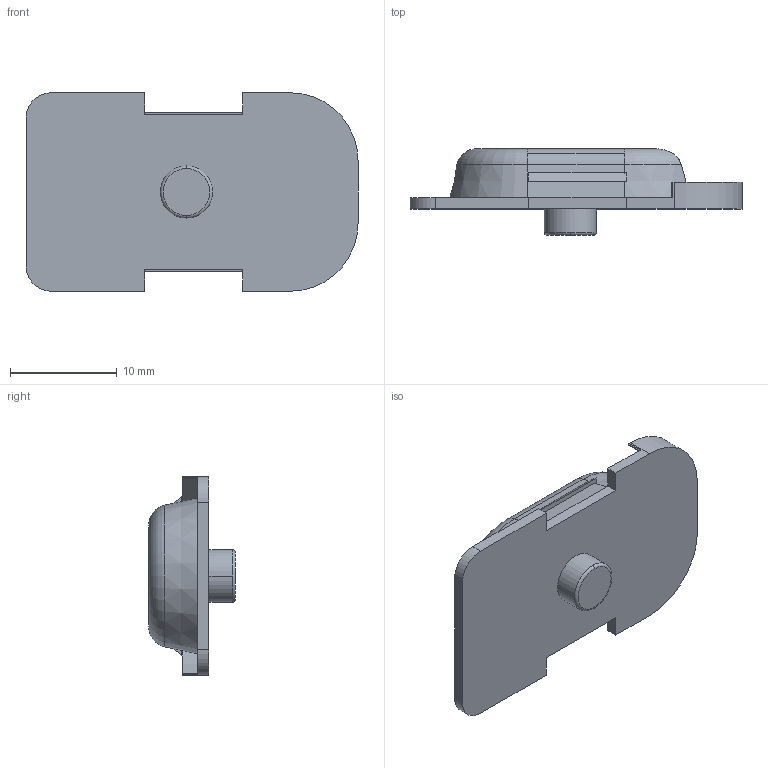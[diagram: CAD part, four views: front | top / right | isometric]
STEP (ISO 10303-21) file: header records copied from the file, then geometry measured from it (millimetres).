
FILE_DESCRIPTION (( 'STEP AP214' ), '1' );
FILE_NAME ('Magazine Insert.step', '2014-07-30T19:46:14', ( 'WarFairy' ), ( '' ), 'SwSTEP 2.0', 'SolidWorks 2013', '' );
FILE_SCHEMA (( 'AUTOMOTIVE_DESIGN' ));
Length unit declared in the file: millimetre
Products named in the file (1): Magazine Insert
Bounding box: 31.1 x 8.1 x 18.59 mm (x, y, z)
Volume: 1309.1 mm3; surface area: 1661.6 mm2
Topology: 1 solids, 1 shells, 70 faces, 189 edges, 122 vertices
Faces by surface type: plane 45, cylinder 18, torus 5, cone 2
Entity records: 2244 total; most frequent: CARTESIAN_POINT 412, DIRECTION 380, ORIENTED_EDGE 378, EDGE_CURVE 189, VECTOR 132, LINE 132, AXIS2_PLACEMENT_3D 124, VERTEX_POINT 122
